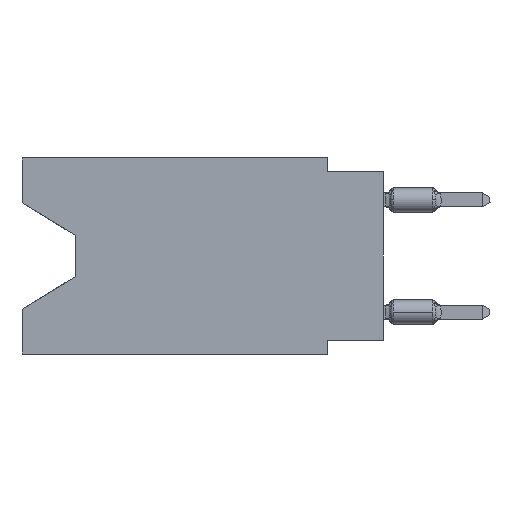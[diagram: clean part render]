
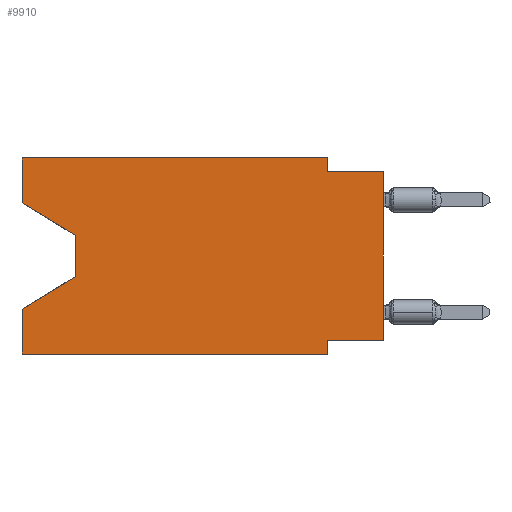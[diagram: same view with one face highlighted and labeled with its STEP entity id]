
A CAD part, left-side view. The second image highlights one B-rep face of the part: STEP entity #9910.
In plain terms, the highlighted planar face has unit normal (-1, 0, 0).
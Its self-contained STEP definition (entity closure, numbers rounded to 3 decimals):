
#158 = VERTEX_POINT ( 'NONE', #185 ) ;
#185 = CARTESIAN_POINT ( 'NONE',  ( 0., 13.97, -3.505 ) ) ;
#485 = VERTEX_POINT ( 'NONE', #7562 ) ;
#488 = VERTEX_POINT ( 'NONE', #4579 ) ;
#603 = VERTEX_POINT ( 'NONE', #6558 ) ;
#722 = VECTOR ( 'NONE', #4471, 1000. ) ;
#1177 = LINE ( 'NONE', #2515, #1546 ) ;
#1195 = DIRECTION ( 'NONE',  ( 0., 0., 1. ) ) ;
#1196 = ORIENTED_EDGE ( 'NONE', *, *, #9071, .T. ) ;
#1546 = VECTOR ( 'NONE', #16003, 1000. ) ;
#1645 = EDGE_CURVE ( 'NONE', #158, #485, #21294, .T. ) ;
#1763 = ORIENTED_EDGE ( 'NONE', *, *, #9949, .F. ) ;
#1837 = CARTESIAN_POINT ( 'NONE',  ( 0., 0., 0. ) ) ;
#1855 = ORIENTED_EDGE ( 'NONE', *, *, #11023, .F. ) ;
#1937 = DIRECTION ( 'NONE',  ( 0., 0., 1. ) ) ;
#2193 = CARTESIAN_POINT ( 'NONE',  ( 0., 0., -8.255 ) ) ;
#2492 = VECTOR ( 'NONE', #20390, 1000. ) ;
#2515 = CARTESIAN_POINT ( 'NONE',  ( 0., 16.383, 0. ) ) ;
#2715 = DIRECTION ( 'NONE',  ( 0., 0., -1. ) ) ;
#2748 = EDGE_CURVE ( 'NONE', #18261, #19481, #16001, .T. ) ;
#2955 = CARTESIAN_POINT ( 'NONE',  ( 0., 2.54, -8.255 ) ) ;
#3106 = ORIENTED_EDGE ( 'NONE', *, *, #6303, .F. ) ;
#3123 = LINE ( 'NONE', #20044, #4505 ) ;
#3157 = CARTESIAN_POINT ( 'NONE',  ( 0., 16.383, 0. ) ) ;
#3860 = CARTESIAN_POINT ( 'NONE',  ( 0., 2.54, -0.635 ) ) ;
#4138 = VECTOR ( 'NONE', #1195, 1000. ) ;
#4440 = VECTOR ( 'NONE', #5069, 1000. ) ;
#4471 = DIRECTION ( 'NONE',  ( 0., 0., -1. ) ) ;
#4505 = VECTOR ( 'NONE', #8431, 1000. ) ;
#4579 = CARTESIAN_POINT ( 'NONE',  ( 0., 16.383, -6.852 ) ) ;
#4986 = VECTOR ( 'NONE', #9696, 1000. ) ;
#5069 = DIRECTION ( 'NONE',  ( 0., 0., -1. ) ) ;
#5311 = ORIENTED_EDGE ( 'NONE', *, *, #16017, .F. ) ;
#5363 = LINE ( 'NONE', #13633, #2492 ) ;
#5821 = DIRECTION ( 'NONE',  ( 0., -1., 0. ) ) ;
#5824 = FACE_OUTER_BOUND ( 'NONE', #18107, .T. ) ;
#6118 = VERTEX_POINT ( 'NONE', #10262 ) ;
#6134 = DIRECTION ( 'NONE',  ( 1., 0., 0. ) ) ;
#6262 = ORIENTED_EDGE ( 'NONE', *, *, #20586, .F. ) ;
#6303 = EDGE_CURVE ( 'NONE', #10734, #7339, #12664, .T. ) ;
#6471 = AXIS2_PLACEMENT_3D ( 'NONE', #7896, #6134, #2715 ) ;
#6558 = CARTESIAN_POINT ( 'NONE',  ( 0., 16.383, -2.038 ) ) ;
#7233 = DIRECTION ( 'NONE',  ( 0., -0.855, -0.519 ) ) ;
#7339 = VERTEX_POINT ( 'NONE', #2955 ) ;
#7562 = CARTESIAN_POINT ( 'NONE',  ( 0., 13.97, -5.385 ) ) ;
#7896 = CARTESIAN_POINT ( 'NONE',  ( 0., 16.383, 0. ) ) ;
#8038 = LINE ( 'NONE', #21228, #4986 ) ;
#8181 = VERTEX_POINT ( 'NONE', #3860 ) ;
#8265 = EDGE_CURVE ( 'NONE', #18261, #488, #12786, .T. ) ;
#8403 = LINE ( 'NONE', #11721, #12852 ) ;
#8431 = DIRECTION ( 'NONE',  ( 0., 0., -1. ) ) ;
#8605 = VECTOR ( 'NONE', #7233, 1000. ) ;
#9071 = EDGE_CURVE ( 'NONE', #10734, #6118, #10231, .T. ) ;
#9696 = DIRECTION ( 'NONE',  ( 0., 0.855, -0.519 ) ) ;
#9804 = ORIENTED_EDGE ( 'NONE', *, *, #1645, .T. ) ;
#9910 = ADVANCED_FACE ( 'NONE', ( #5824 ), #16310, .F. ) ;
#9949 = EDGE_CURVE ( 'NONE', #12449, #14499, #1177, .T. ) ;
#10183 = CARTESIAN_POINT ( 'NONE',  ( 0., 2.54, 0. ) ) ;
#10192 = EDGE_CURVE ( 'NONE', #603, #158, #10237, .T. ) ;
#10231 = LINE ( 'NONE', #1837, #10353 ) ;
#10237 = LINE ( 'NONE', #16988, #8605 ) ;
#10262 = CARTESIAN_POINT ( 'NONE',  ( 0., 0., -0.635 ) ) ;
#10353 = VECTOR ( 'NONE', #1937, 1000. ) ;
#10429 = ORIENTED_EDGE ( 'NONE', *, *, #8265, .F. ) ;
#10734 = VERTEX_POINT ( 'NONE', #10968 ) ;
#10968 = CARTESIAN_POINT ( 'NONE',  ( 0., 0., -8.255 ) ) ;
#11016 = DIRECTION ( 'NONE',  ( 0., 1., 0. ) ) ;
#11023 = EDGE_CURVE ( 'NONE', #8181, #6118, #8403, .T. ) ;
#11595 = ORIENTED_EDGE ( 'NONE', *, *, #17071, .T. ) ;
#11721 = CARTESIAN_POINT ( 'NONE',  ( 0., 0., -0.635 ) ) ;
#12057 = DIRECTION ( 'NONE',  ( 0., -1., 0. ) ) ;
#12449 = VERTEX_POINT ( 'NONE', #3157 ) ;
#12479 = ORIENTED_EDGE ( 'NONE', *, *, #10192, .T. ) ;
#12664 = LINE ( 'NONE', #2193, #20423 ) ;
#12786 = LINE ( 'NONE', #21225, #4138 ) ;
#12842 = EDGE_CURVE ( 'NONE', #7339, #19481, #3123, .T. ) ;
#12852 = VECTOR ( 'NONE', #12057, 1000. ) ;
#13633 = CARTESIAN_POINT ( 'NONE',  ( 0., 16.383, 0. ) ) ;
#14117 = CARTESIAN_POINT ( 'NONE',  ( 0., 16.383, -8.89 ) ) ;
#14499 = VERTEX_POINT ( 'NONE', #10183 ) ;
#14786 = CARTESIAN_POINT ( 'NONE',  ( 0., 16.383, -8.89 ) ) ;
#15135 = CARTESIAN_POINT ( 'NONE',  ( 0., 2.54, -8.89 ) ) ;
#15639 = ORIENTED_EDGE ( 'NONE', *, *, #12842, .F. ) ;
#15732 = VECTOR ( 'NONE', #5821, 1000. ) ;
#16001 = LINE ( 'NONE', #14117, #15732 ) ;
#16003 = DIRECTION ( 'NONE',  ( 0., -1., 0. ) ) ;
#16017 = EDGE_CURVE ( 'NONE', #603, #12449, #5363, .T. ) ;
#16310 = PLANE ( 'NONE',  #6471 ) ;
#16988 = CARTESIAN_POINT ( 'NONE',  ( 0., 16.383, -2.038 ) ) ;
#17071 = EDGE_CURVE ( 'NONE', #485, #488, #8038, .T. ) ;
#17247 = LINE ( 'NONE', #20436, #4440 ) ;
#18107 = EDGE_LOOP ( 'NONE', ( #12479, #9804, #11595, #10429, #18372, #15639, #3106, #1196, #1855, #6262, #1763, #5311 ) ) ;
#18261 = VERTEX_POINT ( 'NONE', #14786 ) ;
#18372 = ORIENTED_EDGE ( 'NONE', *, *, #2748, .T. ) ;
#19481 = VERTEX_POINT ( 'NONE', #15135 ) ;
#20044 = CARTESIAN_POINT ( 'NONE',  ( 0., 2.54, -8.89 ) ) ;
#20390 = DIRECTION ( 'NONE',  ( 0., 0., 1. ) ) ;
#20423 = VECTOR ( 'NONE', #11016, 1000. ) ;
#20436 = CARTESIAN_POINT ( 'NONE',  ( 0., 2.54, 0. ) ) ;
#20586 = EDGE_CURVE ( 'NONE', #14499, #8181, #17247, .T. ) ;
#21225 = CARTESIAN_POINT ( 'NONE',  ( 0., 16.383, 0. ) ) ;
#21228 = CARTESIAN_POINT ( 'NONE',  ( 0., 13.97, -5.385 ) ) ;
#21294 = LINE ( 'NONE', #21397, #722 ) ;
#21397 = CARTESIAN_POINT ( 'NONE',  ( 0., 13.97, -3.505 ) ) ;
